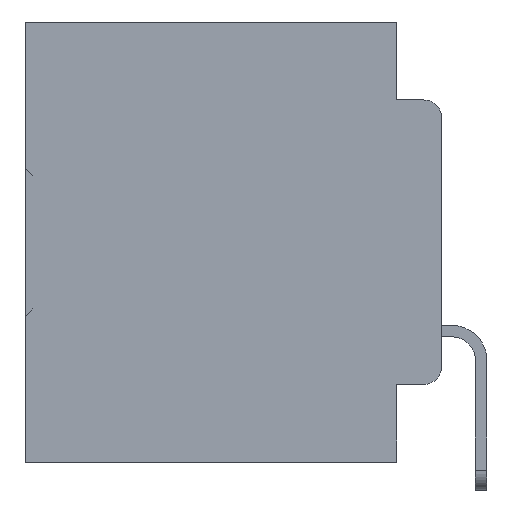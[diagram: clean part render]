
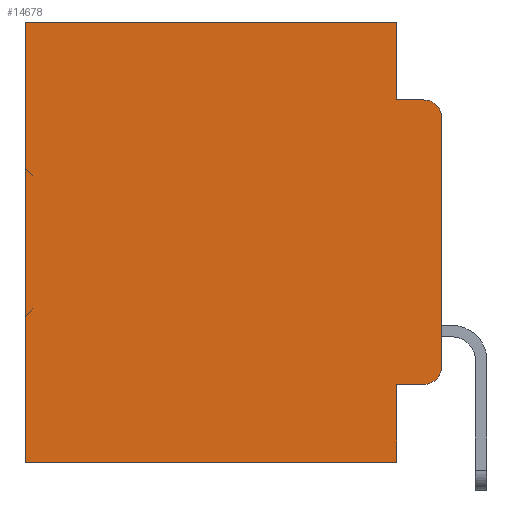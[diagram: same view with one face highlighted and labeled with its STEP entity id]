
A CAD part, left-side view. The second image highlights one B-rep face of the part: STEP entity #14678.
In plain terms, the highlighted planar face has unit normal (-1, 0, 0).
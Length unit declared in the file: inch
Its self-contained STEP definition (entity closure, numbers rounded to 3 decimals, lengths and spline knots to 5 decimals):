
#476 = EDGE_CURVE ( 'NONE', #12299, #32903, #20242, .T. ) ;
#888 = VECTOR ( 'NONE', #27375, 39.37008 ) ;
#1692 = DIRECTION ( 'NONE',  ( 1., 0., 0. ) ) ;
#1870 = LINE ( 'NONE', #24483, #888 ) ;
#2082 = AXIS2_PLACEMENT_3D ( 'NONE', #8697, #28757, #11765 ) ;
#2242 = CARTESIAN_POINT ( 'NONE',  ( 0.298, 0., 0. ) ) ;
#3047 = VERTEX_POINT ( 'NONE', #21392 ) ;
#3649 = CARTESIAN_POINT ( 'NONE',  ( 0.298, 0.051, -0.4115 ) ) ;
#3815 = DIRECTION ( 'NONE',  ( -1., 0., 0. ) ) ;
#4210 = LINE ( 'NONE', #3649, #33717 ) ;
#4343 = EDGE_CURVE ( 'NONE', #6171, #14388, #31046, .T. ) ;
#4761 = CARTESIAN_POINT ( 'NONE',  ( 0.298, 0.473, 0. ) ) ;
#4779 = LINE ( 'NONE', #15110, #35079 ) ;
#6041 = CARTESIAN_POINT ( 'NONE',  ( 0.298, 0.051, 0. ) ) ;
#6171 = VERTEX_POINT ( 'NONE', #28547 ) ;
#6415 = ORIENTED_EDGE ( 'NONE', *, *, #17524, .F. ) ;
#6559 = VECTOR ( 'NONE', #25614, 39.37008 ) ;
#7060 = DIRECTION ( 'NONE',  ( 0., 0., -1. ) ) ;
#7443 = CIRCLE ( 'NONE', #2082, 0.02 ) ;
#7702 = CARTESIAN_POINT ( 'NONE',  ( 0.298, 0., 0. ) ) ;
#8117 = EDGE_CURVE ( 'NONE', #6171, #22425, #25619, .T. ) ;
#8291 = EDGE_CURVE ( 'NONE', #34001, #12299, #4779, .T. ) ;
#8339 = DIRECTION ( 'NONE',  ( 0., 0., -1. ) ) ;
#8572 = EDGE_CURVE ( 'NONE', #3047, #32903, #26468, .T. ) ;
#8697 = CARTESIAN_POINT ( 'NONE',  ( 0.298, 0.02, -0.3915 ) ) ;
#10233 = EDGE_LOOP ( 'NONE', ( #32665, #20493, #36887, #12499, #22280, #24023, #34013, #6415, #16232, #23601 ) ) ;
#10461 = VECTOR ( 'NONE', #8339, 39.37008 ) ;
#10749 = EDGE_CURVE ( 'NONE', #21191, #22425, #7443, .T. ) ;
#10909 = FACE_OUTER_BOUND ( 'NONE', #10233, .T. ) ;
#11765 = DIRECTION ( 'NONE',  ( 0., 0., -1. ) ) ;
#12299 = VERTEX_POINT ( 'NONE', #33559 ) ;
#12499 = ORIENTED_EDGE ( 'NONE', *, *, #22283, .F. ) ;
#12670 = VECTOR ( 'NONE', #7060, 39.37008 ) ;
#14197 = CARTESIAN_POINT ( 'NONE',  ( 0.298, 0.051, 0. ) ) ;
#14388 = VERTEX_POINT ( 'NONE', #21020 ) ;
#14678 = ADVANCED_FACE ( 'NONE', ( #10909 ), #27814, .F. ) ;
#15110 = CARTESIAN_POINT ( 'NONE',  ( 0.298, 0., 0. ) ) ;
#16232 = ORIENTED_EDGE ( 'NONE', *, *, #17806, .T. ) ;
#17054 = DIRECTION ( 'NONE',  ( 0., 1., 0. ) ) ;
#17524 = EDGE_CURVE ( 'NONE', #26491, #3047, #22886, .T. ) ;
#17806 = EDGE_CURVE ( 'NONE', #26491, #21191, #4210, .T. ) ;
#18283 = DIRECTION ( 'NONE',  ( 0., -1., 0. ) ) ;
#19527 = CARTESIAN_POINT ( 'NONE',  ( 0.298, 0., -0.3915 ) ) ;
#20242 = LINE ( 'NONE', #4761, #12670 ) ;
#20493 = ORIENTED_EDGE ( 'NONE', *, *, #4343, .T. ) ;
#21020 = CARTESIAN_POINT ( 'NONE',  ( 0.298, 0.02, -0.0885 ) ) ;
#21191 = VERTEX_POINT ( 'NONE', #33698 ) ;
#21306 = CARTESIAN_POINT ( 'NONE',  ( 0.298, 0.02, -0.1085 ) ) ;
#21392 = CARTESIAN_POINT ( 'NONE',  ( 0.298, 0.051, -0.5 ) ) ;
#22236 = DIRECTION ( 'NONE',  ( 0., 0., -1. ) ) ;
#22280 = ORIENTED_EDGE ( 'NONE', *, *, #8291, .T. ) ;
#22283 = EDGE_CURVE ( 'NONE', #34001, #22781, #1870, .T. ) ;
#22425 = VERTEX_POINT ( 'NONE', #19527 ) ;
#22781 = VERTEX_POINT ( 'NONE', #23967 ) ;
#22886 = LINE ( 'NONE', #14197, #6559 ) ;
#23601 = ORIENTED_EDGE ( 'NONE', *, *, #10749, .T. ) ;
#23967 = CARTESIAN_POINT ( 'NONE',  ( 0.298, 0.051, -0.0885 ) ) ;
#24023 = ORIENTED_EDGE ( 'NONE', *, *, #476, .T. ) ;
#24107 = DIRECTION ( 'NONE',  ( 0., 0., -1. ) ) ;
#24483 = CARTESIAN_POINT ( 'NONE',  ( 0.298, 0.051, 0. ) ) ;
#24947 = CARTESIAN_POINT ( 'NONE',  ( 0.298, 0.051, -0.0885 ) ) ;
#25570 = CARTESIAN_POINT ( 'NONE',  ( 0.298, 0.051, -0.4115 ) ) ;
#25578 = VECTOR ( 'NONE', #17054, 39.37008 ) ;
#25614 = DIRECTION ( 'NONE',  ( 0., 0., -1. ) ) ;
#25619 = LINE ( 'NONE', #2242, #10461 ) ;
#26468 = LINE ( 'NONE', #33676, #25578 ) ;
#26491 = VERTEX_POINT ( 'NONE', #25570 ) ;
#27375 = DIRECTION ( 'NONE',  ( 0., 0., -1. ) ) ;
#27814 = PLANE ( 'NONE',  #30951 ) ;
#28547 = CARTESIAN_POINT ( 'NONE',  ( 0.298, 0., -0.1085 ) ) ;
#28757 = DIRECTION ( 'NONE',  ( -1., 0., 0. ) ) ;
#29602 = LINE ( 'NONE', #24947, #35991 ) ;
#30464 = AXIS2_PLACEMENT_3D ( 'NONE', #21306, #3815, #24107 ) ;
#30951 = AXIS2_PLACEMENT_3D ( 'NONE', #7702, #1692, #22236 ) ;
#31046 = CIRCLE ( 'NONE', #30464, 0.02 ) ;
#32665 = ORIENTED_EDGE ( 'NONE', *, *, #8117, .F. ) ;
#32903 = VERTEX_POINT ( 'NONE', #34488 ) ;
#33296 = DIRECTION ( 'NONE',  ( 0., -1., 0. ) ) ;
#33559 = CARTESIAN_POINT ( 'NONE',  ( 0.298, 0.473, 0. ) ) ;
#33676 = CARTESIAN_POINT ( 'NONE',  ( 0.298, 0., -0.5 ) ) ;
#33698 = CARTESIAN_POINT ( 'NONE',  ( 0.298, 0.02, -0.4115 ) ) ;
#33717 = VECTOR ( 'NONE', #18283, 39.37008 ) ;
#34001 = VERTEX_POINT ( 'NONE', #6041 ) ;
#34013 = ORIENTED_EDGE ( 'NONE', *, *, #8572, .F. ) ;
#34488 = CARTESIAN_POINT ( 'NONE',  ( 0.298, 0.473, -0.5 ) ) ;
#34580 = DIRECTION ( 'NONE',  ( 0., 1., 0. ) ) ;
#35079 = VECTOR ( 'NONE', #34580, 39.37008 ) ;
#35991 = VECTOR ( 'NONE', #33296, 39.37008 ) ;
#36887 = ORIENTED_EDGE ( 'NONE', *, *, #37038, .F. ) ;
#37038 = EDGE_CURVE ( 'NONE', #22781, #14388, #29602, .T. ) ;
